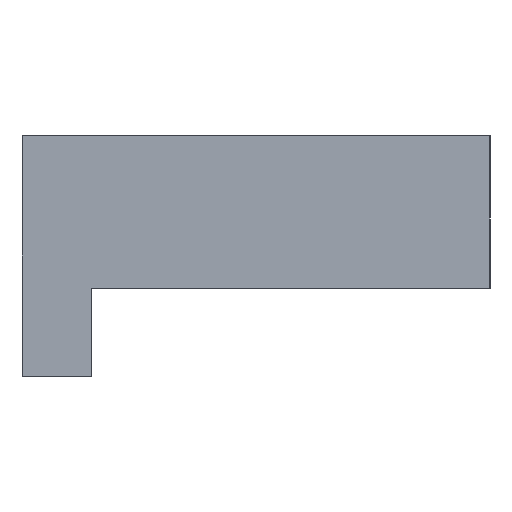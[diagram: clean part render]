
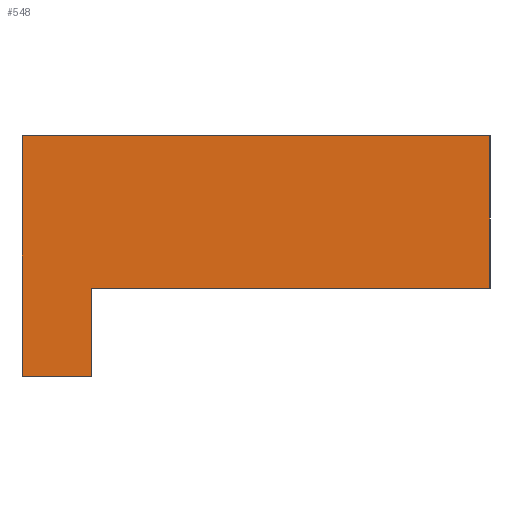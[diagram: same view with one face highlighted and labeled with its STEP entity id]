
A CAD part, left-side view. The second image highlights one B-rep face of the part: STEP entity #548.
In plain terms, the highlighted planar face has unit normal (-1, 0, 0).
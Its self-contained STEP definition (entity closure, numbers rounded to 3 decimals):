
#22=LINE('',#8424,#40);
#23=LINE('',#9073,#41);
#28=LINE('',#9084,#46);
#31=LINE('',#9088,#49);
#34=LINE('',#9095,#52);
#35=LINE('',#9096,#53);
#40=VECTOR('',#622,10.);
#41=VECTOR('',#625,10.);
#46=VECTOR('',#632,10.);
#49=VECTOR('',#637,10.);
#52=VECTOR('',#644,10.);
#53=VECTOR('',#645,10.);
#60=PLANE('',#584);
#80=FACE_OUTER_BOUND('',#98,.T.);
#98=EDGE_LOOP('',(#509,#510,#511,#512,#513,#514));
#243=VERTEX_POINT('',#8417);
#246=VERTEX_POINT('',#8422);
#247=VERTEX_POINT('',#9072);
#251=VERTEX_POINT('',#9081);
#252=VERTEX_POINT('',#9083);
#254=VERTEX_POINT('',#9094);
#328=EDGE_CURVE('',#243,#246,#22,.T.);
#333=EDGE_CURVE('',#243,#247,#23,.T.);
#338=EDGE_CURVE('',#252,#251,#28,.T.);
#341=EDGE_CURVE('',#247,#251,#31,.T.);
#344=EDGE_CURVE('',#254,#246,#34,.T.);
#345=EDGE_CURVE('',#252,#254,#35,.T.);
#509=ORIENTED_EDGE('',*,*,#338,.T.);
#510=ORIENTED_EDGE('',*,*,#341,.F.);
#511=ORIENTED_EDGE('',*,*,#333,.F.);
#512=ORIENTED_EDGE('',*,*,#328,.T.);
#513=ORIENTED_EDGE('',*,*,#344,.F.);
#514=ORIENTED_EDGE('',*,*,#345,.F.);
#548=ADVANCED_FACE('',(#80),#60,.F.);
#584=AXIS2_PLACEMENT_3D('',#9093,#642,#643);
#622=DIRECTION('',(0.,-1.,0.));
#625=DIRECTION('',(0.,0.,-1.));
#632=DIRECTION('',(0.,0.,-1.));
#637=DIRECTION('',(0.,1.,0.));
#642=DIRECTION('center_axis',(1.,0.,0.));
#643=DIRECTION('ref_axis',(0.,-1.,0.));
#644=DIRECTION('',(0.,0.,-1.));
#645=DIRECTION('',(0.,-1.,0.));
#8417=CARTESIAN_POINT('',(2.134,0.84,-10.036));
#8422=CARTESIAN_POINT('',(2.134,-5.782,-10.036));
#8424=CARTESIAN_POINT('',(2.134,1.92,-10.036));
#9072=CARTESIAN_POINT('',(2.134,0.84,-11.5));
#9073=CARTESIAN_POINT('',(2.134,0.84,-9.5));
#9081=CARTESIAN_POINT('',(2.134,2.,-11.5));
#9083=CARTESIAN_POINT('',(2.134,2.,-7.5));
#9084=CARTESIAN_POINT('',(2.134,2.,-7.5));
#9088=CARTESIAN_POINT('',(2.134,-6.875,-11.5));
#9093=CARTESIAN_POINT('Origin',(2.134,2.5,-7.5));
#9094=CARTESIAN_POINT('',(2.134,-5.782,-7.5));
#9095=CARTESIAN_POINT('',(2.134,-5.782,-7.5));
#9096=CARTESIAN_POINT('',(2.134,-6.875,-7.5));
